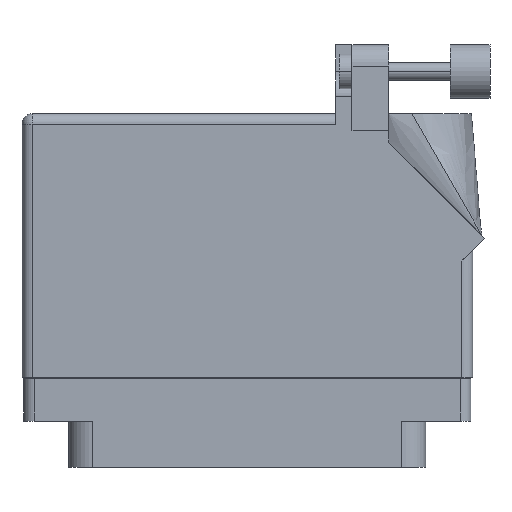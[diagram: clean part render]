
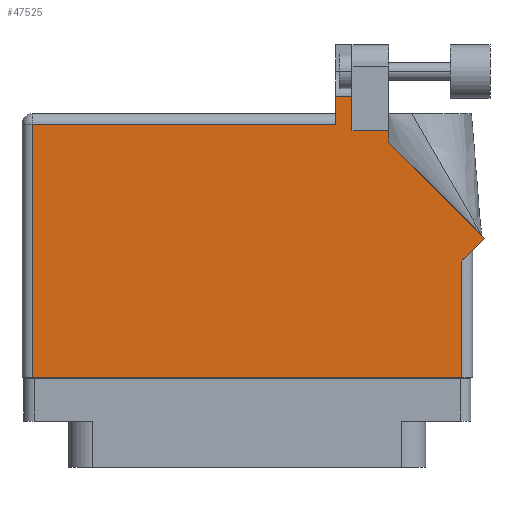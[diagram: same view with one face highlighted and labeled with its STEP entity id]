
A CAD part, front view. The second image highlights one B-rep face of the part: STEP entity #47525.
In plain terms, the highlighted face is planar.
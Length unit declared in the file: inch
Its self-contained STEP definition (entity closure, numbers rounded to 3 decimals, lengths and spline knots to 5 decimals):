
#1129 = CARTESIAN_POINT ( 'NONE',  ( 1.244, 0.575, 0.455 ) ) ;
#1557 = VERTEX_POINT ( 'NONE', #40800 ) ;
#1633 = EDGE_CURVE ( 'NONE', #12313, #2761, #38834, .T. ) ;
#2536 = DIRECTION ( 'NONE',  ( 1., 0., 0. ) ) ;
#2761 = VERTEX_POINT ( 'NONE', #17384 ) ;
#3055 = CARTESIAN_POINT ( 'NONE',  ( -1.244, 1.368, 0.455 ) ) ;
#3655 = VECTOR ( 'NONE', #27335, 39.37008 ) ;
#4578 = CARTESIAN_POINT ( 'NONE',  ( 0.93777, 1.5315, 0.455 ) ) ;
#4858 = EDGE_CURVE ( 'NONE', #28867, #1557, #25797, .T. ) ;
#5009 = LINE ( 'NONE', #4578, #7333 ) ;
#5147 = CARTESIAN_POINT ( 'NONE',  ( 1.37671, 0.70771, 0.455 ) ) ;
#5855 = VECTOR ( 'NONE', #8532, 39.37008 ) ;
#6440 = ORIENTED_EDGE ( 'NONE', *, *, #35236, .T. ) ;
#6559 = VERTEX_POINT ( 'NONE', #21605 ) ;
#7333 = VECTOR ( 'NONE', #11792, 39.37008 ) ;
#8437 = ORIENTED_EDGE ( 'NONE', *, *, #16795, .T. ) ;
#8532 = DIRECTION ( 'NONE',  ( -0.707, 0.707, 0. ) ) ;
#9022 = VECTOR ( 'NONE', #19459, 39.37008 ) ;
#9810 = EDGE_CURVE ( 'NONE', #11666, #6559, #37318, .T. ) ;
#10047 = ORIENTED_EDGE ( 'NONE', *, *, #39472, .T. ) ;
#10352 = ORIENTED_EDGE ( 'NONE', *, *, #28341, .T. ) ;
#11666 = VERTEX_POINT ( 'NONE', #37986 ) ;
#11675 = VECTOR ( 'NONE', #12773, 39.37008 ) ;
#11792 = DIRECTION ( 'NONE',  ( -1., 0., 0. ) ) ;
#12313 = VERTEX_POINT ( 'NONE', #1129 ) ;
#12480 = DIRECTION ( 'NONE',  ( 0.707, 0.707, 0. ) ) ;
#12563 = DIRECTION ( 'NONE',  ( -1., 0., 0. ) ) ;
#12773 = DIRECTION ( 'NONE',  ( -1., 0., 0. ) ) ;
#14089 = VERTEX_POINT ( 'NONE', #14952 ) ;
#14430 = ORIENTED_EDGE ( 'NONE', *, *, #1633, .T. ) ;
#14952 = CARTESIAN_POINT ( 'NONE',  ( -1.244, -0.1, 0.455 ) ) ;
#15701 = LINE ( 'NONE', #5147, #5855 ) ;
#15905 = ORIENTED_EDGE ( 'NONE', *, *, #16052, .T. ) ;
#16052 = EDGE_CURVE ( 'NONE', #2761, #11666, #15701, .T. ) ;
#16133 = FACE_OUTER_BOUND ( 'NONE', #45508, .T. ) ;
#16295 = LINE ( 'NONE', #39583, #41095 ) ;
#16728 = CARTESIAN_POINT ( 'NONE',  ( -1.306, 1.368, 0.455 ) ) ;
#16795 = EDGE_CURVE ( 'NONE', #6559, #17770, #17330, .T. ) ;
#17330 = LINE ( 'NONE', #41809, #21399 ) ;
#17384 = CARTESIAN_POINT ( 'NONE',  ( 1.37671, 0.70771, 0.455 ) ) ;
#17575 = DIRECTION ( 'NONE',  ( -1., 0., 0. ) ) ;
#17770 = VERTEX_POINT ( 'NONE', #40642 ) ;
#18063 = LINE ( 'NONE', #16728, #11675 ) ;
#18109 = VECTOR ( 'NONE', #12480, 39.37008 ) ;
#18329 = CARTESIAN_POINT ( 'NONE',  ( 1.244, 0.637, 0.455 ) ) ;
#19282 = ORIENTED_EDGE ( 'NONE', *, *, #9810, .T. ) ;
#19418 = VECTOR ( 'NONE', #2536, 39.37008 ) ;
#19459 = DIRECTION ( 'NONE',  ( 0., 1., 0. ) ) ;
#20251 = CARTESIAN_POINT ( 'NONE',  ( 0.607, 1.33, 0.455 ) ) ;
#21399 = VECTOR ( 'NONE', #12563, 39.37008 ) ;
#21605 = CARTESIAN_POINT ( 'NONE',  ( 0.82, 1.33, 0.455 ) ) ;
#21943 = CARTESIAN_POINT ( 'NONE',  ( 1.244, -0.1, 0.455 ) ) ;
#22263 = EDGE_CURVE ( 'NONE', #29514, #28867, #5009, .T. ) ;
#23274 = LINE ( 'NONE', #20251, #3655 ) ;
#23527 = ORIENTED_EDGE ( 'NONE', *, *, #4858, .T. ) ;
#24792 = DIRECTION ( 'NONE',  ( 0., -1., 0. ) ) ;
#25797 = LINE ( 'NONE', #43414, #28582 ) ;
#25931 = DIRECTION ( 'NONE',  ( 0., 1., 0. ) ) ;
#27317 = CARTESIAN_POINT ( 'NONE',  ( 0.513, 1.5315, 0.455 ) ) ;
#27335 = DIRECTION ( 'NONE',  ( 0., 1., 0. ) ) ;
#27560 = CARTESIAN_POINT ( 'NONE',  ( 1.306, 0.637, 0.455 ) ) ;
#28341 = EDGE_CURVE ( 'NONE', #1557, #32161, #18063, .T. ) ;
#28582 = VECTOR ( 'NONE', #28875, 39.37008 ) ;
#28807 = CARTESIAN_POINT ( 'NONE',  ( -1.306, 1.43, 0.455 ) ) ;
#28867 = VERTEX_POINT ( 'NONE', #27317 ) ;
#28875 = DIRECTION ( 'NONE',  ( 0., -1., 0. ) ) ;
#29122 = ORIENTED_EDGE ( 'NONE', *, *, #38104, .T. ) ;
#29514 = VERTEX_POINT ( 'NONE', #30977 ) ;
#30977 = CARTESIAN_POINT ( 'NONE',  ( 0.607, 1.5315, 0.455 ) ) ;
#31400 = CARTESIAN_POINT ( 'NONE',  ( -1.306, -0.1, 0.455 ) ) ;
#31687 = LINE ( 'NONE', #18329, #42635 ) ;
#32161 = VERTEX_POINT ( 'NONE', #3055 ) ;
#32343 = VERTEX_POINT ( 'NONE', #21943 ) ;
#32860 = DIRECTION ( 'NONE',  ( 0., 0., -1. ) ) ;
#33490 = ORIENTED_EDGE ( 'NONE', *, *, #33539, .T. ) ;
#33539 = EDGE_CURVE ( 'NONE', #14089, #32343, #36146, .T. ) ;
#34691 = CARTESIAN_POINT ( 'NONE',  ( 0.82, 1.26442, 0.455 ) ) ;
#35236 = EDGE_CURVE ( 'NONE', #17770, #29514, #23274, .T. ) ;
#36146 = LINE ( 'NONE', #31400, #19418 ) ;
#36560 = PLANE ( 'NONE',  #38840 ) ;
#37318 = LINE ( 'NONE', #34691, #9022 ) ;
#37986 = CARTESIAN_POINT ( 'NONE',  ( 0.82, 1.26442, 0.455 ) ) ;
#38104 = EDGE_CURVE ( 'NONE', #32161, #14089, #16295, .T. ) ;
#38834 = LINE ( 'NONE', #27560, #18109 ) ;
#38840 = AXIS2_PLACEMENT_3D ( 'NONE', #28807, #32860, #17575 ) ;
#39472 = EDGE_CURVE ( 'NONE', #32343, #12313, #31687, .T. ) ;
#39583 = CARTESIAN_POINT ( 'NONE',  ( -1.244, -0.1, 0.455 ) ) ;
#40642 = CARTESIAN_POINT ( 'NONE',  ( 0.607, 1.33, 0.455 ) ) ;
#40800 = CARTESIAN_POINT ( 'NONE',  ( 0.513, 1.368, 0.455 ) ) ;
#41095 = VECTOR ( 'NONE', #24792, 39.37008 ) ;
#41809 = CARTESIAN_POINT ( 'NONE',  ( 0.82, 1.33, 0.455 ) ) ;
#42635 = VECTOR ( 'NONE', #25931, 39.37008 ) ;
#43142 = ORIENTED_EDGE ( 'NONE', *, *, #22263, .T. ) ;
#43414 = CARTESIAN_POINT ( 'NONE',  ( 0.513, 1.43, 0.455 ) ) ;
#45508 = EDGE_LOOP ( 'NONE', ( #6440, #43142, #23527, #10352, #29122, #33490, #10047, #14430, #15905, #19282, #8437 ) ) ;
#47525 = ADVANCED_FACE ( 'NONE', ( #16133 ), #36560, .F. ) ;
